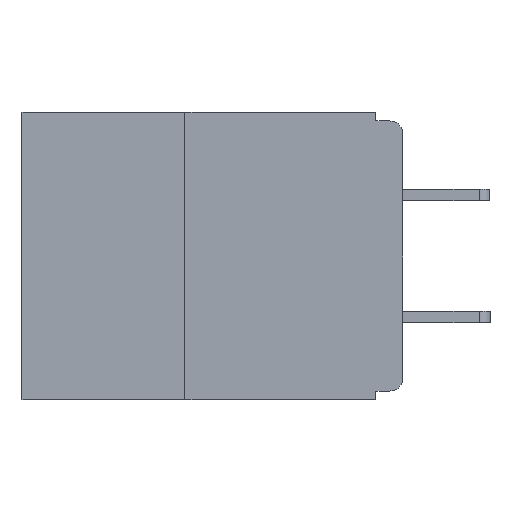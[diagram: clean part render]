
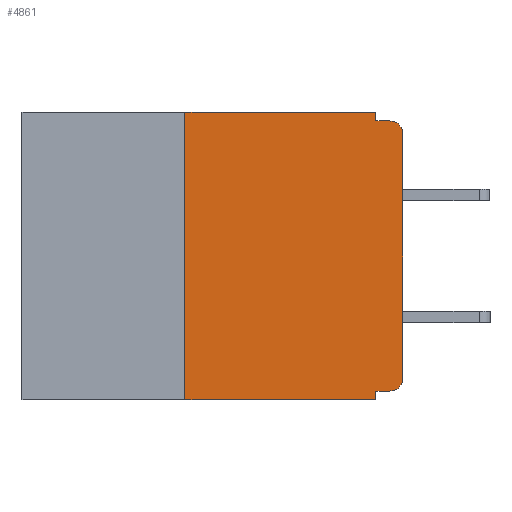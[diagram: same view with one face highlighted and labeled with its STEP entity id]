
A CAD part, left-side view. The second image highlights one B-rep face of the part: STEP entity #4861.
In plain terms, the highlighted planar face has unit normal (-1, 0, 0).
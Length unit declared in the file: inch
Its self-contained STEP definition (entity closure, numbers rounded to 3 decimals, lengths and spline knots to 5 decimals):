
#1296 = DIRECTION ( 'NONE',  ( -1., 0., 0. ) ) ;
#1717 = FACE_OUTER_BOUND ( 'NONE', #9180, .T. ) ;
#2166 = DIRECTION ( 'NONE',  ( 0., 0., -1. ) ) ;
#2562 = EDGE_CURVE ( 'NONE', #17033, #11001, #24401, .T. ) ;
#2651 = DIRECTION ( 'NONE',  ( 0., 0., 1. ) ) ;
#2767 = CARTESIAN_POINT ( 'NONE',  ( 0., 0.25, -0.33 ) ) ;
#2897 = ORIENTED_EDGE ( 'NONE', *, *, #14348, .T. ) ;
#3132 = VECTOR ( 'NONE', #24029, 39.37008 ) ;
#3376 = VERTEX_POINT ( 'NONE', #14738 ) ;
#4075 = CARTESIAN_POINT ( 'NONE',  ( 0., 0., -0.01 ) ) ;
#4525 = VECTOR ( 'NONE', #11134, 39.37008 ) ;
#4861 = ADVANCED_FACE ( 'NONE', ( #1717 ), #20034, .F. ) ;
#5743 = CARTESIAN_POINT ( 'NONE',  ( 0., 0.437, 0. ) ) ;
#5792 = CARTESIAN_POINT ( 'NONE',  ( 0., 0.031, -0.32 ) ) ;
#5898 = EDGE_CURVE ( 'NONE', #24126, #9320, #28529, .T. ) ;
#6596 = CARTESIAN_POINT ( 'NONE',  ( 0., 0.015, -0.025 ) ) ;
#6739 = CARTESIAN_POINT ( 'NONE',  ( 0., 0.25, 0. ) ) ;
#7038 = CARTESIAN_POINT ( 'NONE',  ( 0., 0.031, 0. ) ) ;
#7127 = VERTEX_POINT ( 'NONE', #8407 ) ;
#7370 = CARTESIAN_POINT ( 'NONE',  ( 0., 0., -0.32 ) ) ;
#7392 = VERTEX_POINT ( 'NONE', #7038 ) ;
#7498 = CARTESIAN_POINT ( 'NONE',  ( 0., 0.031, -0.01 ) ) ;
#8084 = CARTESIAN_POINT ( 'NONE',  ( 0., 0.437, 0. ) ) ;
#8146 = DIRECTION ( 'NONE',  ( 1., 0., 0. ) ) ;
#8407 = CARTESIAN_POINT ( 'NONE',  ( 0., 0.015, -0.32 ) ) ;
#8726 = CARTESIAN_POINT ( 'NONE',  ( 0., 0.031, 0. ) ) ;
#9027 = DIRECTION ( 'NONE',  ( 0., 0., -1. ) ) ;
#9180 = EDGE_LOOP ( 'NONE', ( #2897, #14613, #12885, #19405, #16830, #11181, #13619, #9542, #10972, #12250 ) ) ;
#9320 = VERTEX_POINT ( 'NONE', #14809 ) ;
#9542 = ORIENTED_EDGE ( 'NONE', *, *, #22311, .F. ) ;
#10030 = CIRCLE ( 'NONE', #27465, 0.015 ) ;
#10184 = LINE ( 'NONE', #29944, #10907 ) ;
#10907 = VECTOR ( 'NONE', #11430, 39.37008 ) ;
#10972 = ORIENTED_EDGE ( 'NONE', *, *, #21842, .F. ) ;
#11001 = VERTEX_POINT ( 'NONE', #6739 ) ;
#11134 = DIRECTION ( 'NONE',  ( 0., 0., -1. ) ) ;
#11181 = ORIENTED_EDGE ( 'NONE', *, *, #2562, .F. ) ;
#11344 = EDGE_CURVE ( 'NONE', #7127, #3376, #10030, .T. ) ;
#11430 = DIRECTION ( 'NONE',  ( 0., 0., 1. ) ) ;
#12083 = LINE ( 'NONE', #4075, #23870 ) ;
#12250 = ORIENTED_EDGE ( 'NONE', *, *, #11344, .T. ) ;
#12885 = ORIENTED_EDGE ( 'NONE', *, *, #22818, .F. ) ;
#13599 = VECTOR ( 'NONE', #2166, 39.37008 ) ;
#13619 = ORIENTED_EDGE ( 'NONE', *, *, #26882, .T. ) ;
#13684 = LINE ( 'NONE', #8084, #19297 ) ;
#14137 = AXIS2_PLACEMENT_3D ( 'NONE', #6596, #23195, #9027 ) ;
#14166 = VERTEX_POINT ( 'NONE', #29367 ) ;
#14348 = EDGE_CURVE ( 'NONE', #3376, #24126, #10184, .T. ) ;
#14613 = ORIENTED_EDGE ( 'NONE', *, *, #5898, .T. ) ;
#14738 = CARTESIAN_POINT ( 'NONE',  ( 0., 0., -0.305 ) ) ;
#14809 = CARTESIAN_POINT ( 'NONE',  ( 0., 0.015, -0.01 ) ) ;
#15753 = CARTESIAN_POINT ( 'NONE',  ( 0., 0.015, -0.305 ) ) ;
#16534 = LINE ( 'NONE', #8726, #4525 ) ;
#16830 = ORIENTED_EDGE ( 'NONE', *, *, #27763, .F. ) ;
#17033 = VERTEX_POINT ( 'NONE', #29575 ) ;
#17063 = EDGE_CURVE ( 'NONE', #7392, #28880, #16534, .T. ) ;
#18165 = DIRECTION ( 'NONE',  ( 0., 0., -1. ) ) ;
#18276 = VECTOR ( 'NONE', #2651, 39.37008 ) ;
#18883 = VERTEX_POINT ( 'NONE', #5792 ) ;
#19297 = VECTOR ( 'NONE', #24678, 39.37008 ) ;
#19405 = ORIENTED_EDGE ( 'NONE', *, *, #17063, .F. ) ;
#19931 = LINE ( 'NONE', #30251, #13599 ) ;
#20034 = PLANE ( 'NONE',  #25828 ) ;
#21842 = EDGE_CURVE ( 'NONE', #7127, #18883, #28125, .T. ) ;
#22311 = EDGE_CURVE ( 'NONE', #18883, #14166, #19931, .T. ) ;
#22818 = EDGE_CURVE ( 'NONE', #28880, #9320, #12083, .T. ) ;
#23195 = DIRECTION ( 'NONE',  ( -1., 0., 0. ) ) ;
#23358 = CARTESIAN_POINT ( 'NONE',  ( 0., 0.437, -0.33 ) ) ;
#23645 = VECTOR ( 'NONE', #25627, 39.37008 ) ;
#23870 = VECTOR ( 'NONE', #27496, 39.37008 ) ;
#24029 = DIRECTION ( 'NONE',  ( 0., 1., 0. ) ) ;
#24126 = VERTEX_POINT ( 'NONE', #25288 ) ;
#24347 = LINE ( 'NONE', #23358, #23645 ) ;
#24401 = LINE ( 'NONE', #2767, #18276 ) ;
#24644 = DIRECTION ( 'NONE',  ( 0., 0., -1. ) ) ;
#24678 = DIRECTION ( 'NONE',  ( 0., -1., 0. ) ) ;
#25288 = CARTESIAN_POINT ( 'NONE',  ( 0., 0., -0.025 ) ) ;
#25627 = DIRECTION ( 'NONE',  ( 0., -1., 0. ) ) ;
#25828 = AXIS2_PLACEMENT_3D ( 'NONE', #5743, #8146, #24644 ) ;
#26882 = EDGE_CURVE ( 'NONE', #17033, #14166, #24347, .T. ) ;
#27465 = AXIS2_PLACEMENT_3D ( 'NONE', #15753, #1296, #18165 ) ;
#27496 = DIRECTION ( 'NONE',  ( 0., -1., 0. ) ) ;
#27763 = EDGE_CURVE ( 'NONE', #11001, #7392, #13684, .T. ) ;
#28125 = LINE ( 'NONE', #7370, #3132 ) ;
#28529 = CIRCLE ( 'NONE', #14137, 0.015 ) ;
#28880 = VERTEX_POINT ( 'NONE', #7498 ) ;
#29367 = CARTESIAN_POINT ( 'NONE',  ( 0., 0.031, -0.33 ) ) ;
#29575 = CARTESIAN_POINT ( 'NONE',  ( 0., 0.25, -0.33 ) ) ;
#29944 = CARTESIAN_POINT ( 'NONE',  ( 0., 0., 0. ) ) ;
#30251 = CARTESIAN_POINT ( 'NONE',  ( 0., 0.031, -0.33 ) ) ;
